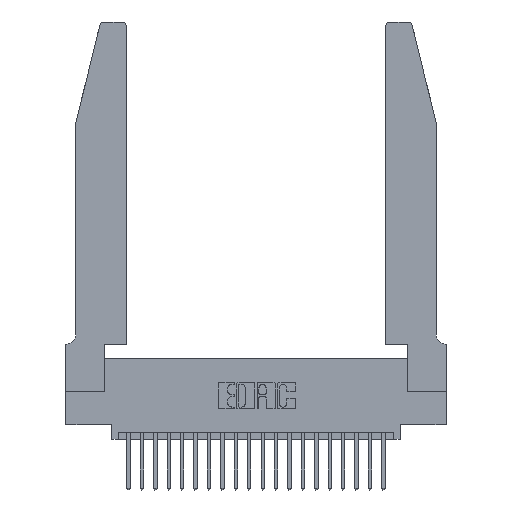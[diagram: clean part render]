
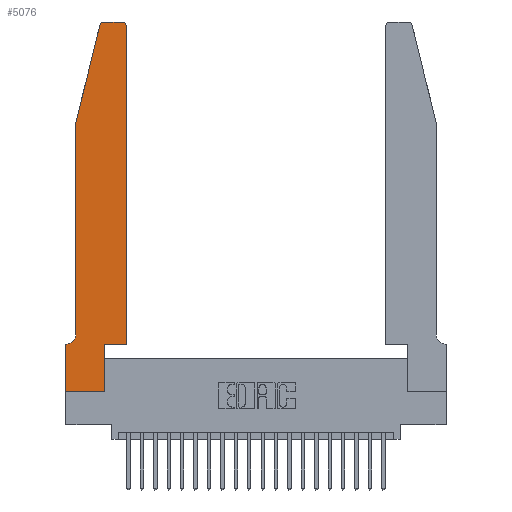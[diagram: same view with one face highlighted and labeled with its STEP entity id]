
A CAD part, top view. The second image highlights one B-rep face of the part: STEP entity #5076.
In plain terms, the highlighted planar face has unit normal (0, 0, 1).
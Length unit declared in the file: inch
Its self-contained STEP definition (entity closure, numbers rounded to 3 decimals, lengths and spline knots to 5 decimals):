
#369 = ORIENTED_EDGE ( 'NONE', *, *, #22643, .T. ) ;
#623 = ORIENTED_EDGE ( 'NONE', *, *, #13736, .T. ) ;
#742 = VECTOR ( 'NONE', #6203, 39.37008 ) ;
#1007 = FACE_OUTER_BOUND ( 'NONE', #22626, .T. ) ;
#1817 = EDGE_CURVE ( 'NONE', #19894, #15394, #17835, .T. ) ;
#2321 = EDGE_CURVE ( 'NONE', #5634, #14420, #7859, .T. ) ;
#2530 = ORIENTED_EDGE ( 'NONE', *, *, #2321, .T. ) ;
#2557 = CARTESIAN_POINT ( 'NONE',  ( 0.0755, 2., 0.37 ) ) ;
#2562 = CARTESIAN_POINT ( 'NONE',  ( 0., 0., 0.37 ) ) ;
#2728 = VECTOR ( 'NONE', #6459, 39.37008 ) ;
#2803 = CARTESIAN_POINT ( 'NONE',  ( 0.0755, 0.35, 0.37 ) ) ;
#2972 = DIRECTION ( 'NONE',  ( -1., 0., 0. ) ) ;
#2996 = DIRECTION ( 'NONE',  ( 0., -1., 0. ) ) ;
#3194 = ORIENTED_EDGE ( 'NONE', *, *, #13772, .T. ) ;
#3442 = DIRECTION ( 'NONE',  ( 0., 1., 0. ) ) ;
#3741 = DIRECTION ( 'NONE',  ( 0., 1., 0. ) ) ;
#4149 = CARTESIAN_POINT ( 'NONE',  ( 0., 0.35, 0.37 ) ) ;
#4152 = VERTEX_POINT ( 'NONE', #18911 ) ;
#4222 = VECTOR ( 'NONE', #11409, 39.37008 ) ;
#4232 = DIRECTION ( 'NONE',  ( 0., 0., 1. ) ) ;
#4303 = DIRECTION ( 'NONE',  ( 0., 0., -1. ) ) ;
#4328 = VERTEX_POINT ( 'NONE', #2557 ) ;
#4783 = LINE ( 'NONE', #15065, #4222 ) ;
#4823 = CARTESIAN_POINT ( 'NONE',  ( 0.0055, 0.35, 0.37 ) ) ;
#5076 = ADVANCED_FACE ( 'NONE', ( #1007 ), #19191, .T. ) ;
#5634 = VERTEX_POINT ( 'NONE', #11945 ) ;
#5794 = ORIENTED_EDGE ( 'NONE', *, *, #21704, .T. ) ;
#6048 = VECTOR ( 'NONE', #3442, 39.37008 ) ;
#6188 = LINE ( 'NONE', #17551, #20175 ) ;
#6203 = DIRECTION ( 'NONE',  ( 0., -1., 0. ) ) ;
#6390 = ORIENTED_EDGE ( 'NONE', *, *, #11235, .T. ) ;
#6459 = DIRECTION ( 'NONE',  ( -1., 0., 0. ) ) ;
#6616 = CARTESIAN_POINT ( 'NONE',  ( 0.4205, 2.72, 0.37 ) ) ;
#6904 = VERTEX_POINT ( 'NONE', #15166 ) ;
#6915 = DIRECTION ( 'NONE',  ( 1., 0., 0. ) ) ;
#7041 = ORIENTED_EDGE ( 'NONE', *, *, #1817, .T. ) ;
#7270 = VECTOR ( 'NONE', #3741, 39.37008 ) ;
#7293 = CIRCLE ( 'NONE', #21169, 0.03 ) ;
#7859 = LINE ( 'NONE', #7946, #16412 ) ;
#7946 = CARTESIAN_POINT ( 'NONE',  ( 0., 0., 0.37 ) ) ;
#8234 = CARTESIAN_POINT ( 'NONE',  ( 0., 0.35, 0.37 ) ) ;
#8470 = DIRECTION ( 'NONE',  ( 1., 0., 0. ) ) ;
#9029 = CARTESIAN_POINT ( 'NONE',  ( 0.0755, 0.42, 0.37 ) ) ;
#9334 = EDGE_CURVE ( 'NONE', #16938, #4328, #4783, .T. ) ;
#10079 = DIRECTION ( 'NONE',  ( 1., 0., 0. ) ) ;
#10270 = CARTESIAN_POINT ( 'NONE',  ( 0.25487, 2.72718, 0.37 ) ) ;
#10560 = CARTESIAN_POINT ( 'NONE',  ( 0.2865, 0., 0.37 ) ) ;
#10894 = LINE ( 'NONE', #19783, #6048 ) ;
#10970 = CARTESIAN_POINT ( 'NONE',  ( 0.4505, 0.35, 0.37 ) ) ;
#11036 = CIRCLE ( 'NONE', #13049, 0.03 ) ;
#11235 = EDGE_CURVE ( 'NONE', #23183, #17594, #22511, .T. ) ;
#11409 = DIRECTION ( 'NONE',  ( -0.239, -0.971, 0. ) ) ;
#11945 = CARTESIAN_POINT ( 'NONE',  ( 0., 0., 0.37 ) ) ;
#12097 = CIRCLE ( 'NONE', #16633, 0.07 ) ;
#12130 = LINE ( 'NONE', #10970, #7270 ) ;
#12680 = ORIENTED_EDGE ( 'NONE', *, *, #21707, .T. ) ;
#12703 = VERTEX_POINT ( 'NONE', #13249 ) ;
#13049 = AXIS2_PLACEMENT_3D ( 'NONE', #6616, #19412, #8470 ) ;
#13249 = CARTESIAN_POINT ( 'NONE',  ( 0.284, 2.75, 0.37 ) ) ;
#13258 = LINE ( 'NONE', #17655, #22403 ) ;
#13368 = VECTOR ( 'NONE', #6915, 39.37008 ) ;
#13736 = EDGE_CURVE ( 'NONE', #18939, #19894, #12097, .T. ) ;
#13772 = EDGE_CURVE ( 'NONE', #15394, #5634, #15238, .T. ) ;
#14387 = ORIENTED_EDGE ( 'NONE', *, *, #9334, .T. ) ;
#14420 = VERTEX_POINT ( 'NONE', #10560 ) ;
#14435 = ORIENTED_EDGE ( 'NONE', *, *, #23093, .T. ) ;
#15065 = CARTESIAN_POINT ( 'NONE',  ( 0.0755, 2., 0.37 ) ) ;
#15093 = EDGE_CURVE ( 'NONE', #14420, #23183, #10894, .T. ) ;
#15133 = CARTESIAN_POINT ( 'NONE',  ( 0.284, 2.72, 0.37 ) ) ;
#15166 = CARTESIAN_POINT ( 'NONE',  ( 0.4205, 2.75, 0.37 ) ) ;
#15206 = CARTESIAN_POINT ( 'NONE',  ( 0.0055, 0.42, 0.37 ) ) ;
#15238 = LINE ( 'NONE', #2562, #742 ) ;
#15394 = VERTEX_POINT ( 'NONE', #4149 ) ;
#15422 = AXIS2_PLACEMENT_3D ( 'NONE', #8234, #21001, #10079 ) ;
#16089 = CARTESIAN_POINT ( 'NONE',  ( 0.4505, 0.35, 0.37 ) ) ;
#16412 = VECTOR ( 'NONE', #18904, 39.37008 ) ;
#16633 = AXIS2_PLACEMENT_3D ( 'NONE', #15206, #4303, #17047 ) ;
#16938 = VERTEX_POINT ( 'NONE', #10270 ) ;
#16971 = DIRECTION ( 'NONE',  ( 1., 0., 0. ) ) ;
#17047 = DIRECTION ( 'NONE',  ( -1., 0., 0. ) ) ;
#17551 = CARTESIAN_POINT ( 'NONE',  ( 0.2605, 2.75, 0.37 ) ) ;
#17594 = VERTEX_POINT ( 'NONE', #19661 ) ;
#17655 = CARTESIAN_POINT ( 'NONE',  ( 0.0755, 2., 0.37 ) ) ;
#17835 = LINE ( 'NONE', #2803, #2728 ) ;
#17848 = ORIENTED_EDGE ( 'NONE', *, *, #22135, .T. ) ;
#18904 = DIRECTION ( 'NONE',  ( 1., 0., 0. ) ) ;
#18911 = CARTESIAN_POINT ( 'NONE',  ( 0.4505, 2.72, 0.37 ) ) ;
#18939 = VERTEX_POINT ( 'NONE', #9029 ) ;
#19191 = PLANE ( 'NONE',  #15422 ) ;
#19412 = DIRECTION ( 'NONE',  ( 0., 0., 1. ) ) ;
#19661 = CARTESIAN_POINT ( 'NONE',  ( 0.4505, 0.35, 0.37 ) ) ;
#19783 = CARTESIAN_POINT ( 'NONE',  ( 0.2865, 0.35, 0.37 ) ) ;
#19894 = VERTEX_POINT ( 'NONE', #4823 ) ;
#20175 = VECTOR ( 'NONE', #2972, 39.37008 ) ;
#20604 = ORIENTED_EDGE ( 'NONE', *, *, #15093, .T. ) ;
#21001 = DIRECTION ( 'NONE',  ( 0., 0., 1. ) ) ;
#21169 = AXIS2_PLACEMENT_3D ( 'NONE', #15133, #4232, #16971 ) ;
#21704 = EDGE_CURVE ( 'NONE', #4152, #6904, #11036, .T. ) ;
#21707 = EDGE_CURVE ( 'NONE', #6904, #12703, #6188, .T. ) ;
#22135 = EDGE_CURVE ( 'NONE', #12703, #16938, #7293, .T. ) ;
#22403 = VECTOR ( 'NONE', #2996, 39.37008 ) ;
#22511 = LINE ( 'NONE', #16089, #13368 ) ;
#22626 = EDGE_LOOP ( 'NONE', ( #12680, #17848, #14387, #14435, #623, #7041, #3194, #2530, #20604, #6390, #369, #5794 ) ) ;
#22643 = EDGE_CURVE ( 'NONE', #17594, #4152, #12130, .T. ) ;
#23093 = EDGE_CURVE ( 'NONE', #4328, #18939, #13258, .T. ) ;
#23183 = VERTEX_POINT ( 'NONE', #23406 ) ;
#23406 = CARTESIAN_POINT ( 'NONE',  ( 0.2865, 0.35, 0.37 ) ) ;
